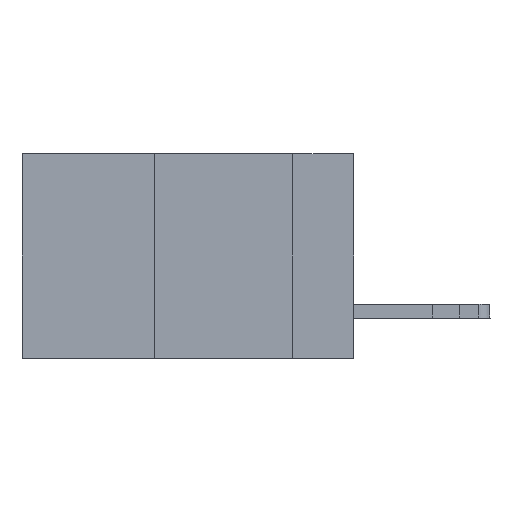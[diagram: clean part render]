
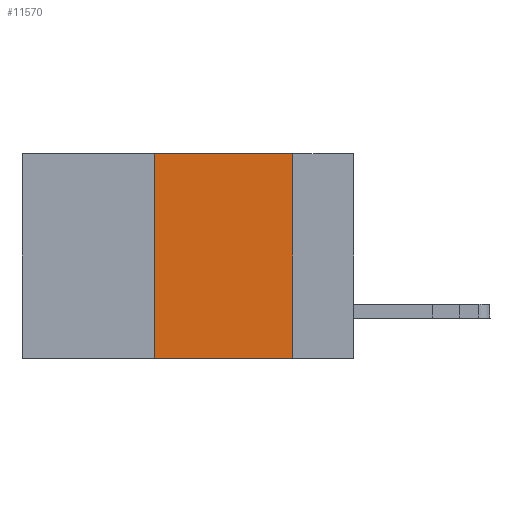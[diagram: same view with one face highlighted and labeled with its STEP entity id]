
A CAD part, left-side view. The second image highlights one B-rep face of the part: STEP entity #11570.
In plain terms, the highlighted planar face has unit normal (-1, 0, 0).
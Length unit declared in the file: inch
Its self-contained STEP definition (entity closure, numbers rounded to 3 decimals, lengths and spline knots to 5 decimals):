
#340 = CARTESIAN_POINT ( 'NONE',  ( 0., 0.36, 0. ) ) ;
#1630 = CARTESIAN_POINT ( 'NONE',  ( 0., 0.6, -0.37 ) ) ;
#2541 = CARTESIAN_POINT ( 'NONE',  ( 0., 0.36, -0.37 ) ) ;
#2728 = LINE ( 'NONE', #13764, #15780 ) ;
#3013 = DIRECTION ( 'NONE',  ( 0., -1., 0. ) ) ;
#3130 = LINE ( 'NONE', #1630, #9951 ) ;
#3228 = EDGE_CURVE ( 'NONE', #16537, #3969, #11790, .T. ) ;
#3969 = VERTEX_POINT ( 'NONE', #9981 ) ;
#5041 = AXIS2_PLACEMENT_3D ( 'NONE', #12373, #7009, #16317 ) ;
#5202 = ORIENTED_EDGE ( 'NONE', *, *, #9447, .F. ) ;
#6876 = CARTESIAN_POINT ( 'NONE',  ( 0., 0.6, 0. ) ) ;
#7009 = DIRECTION ( 'NONE',  ( 1., 0., 0. ) ) ;
#7068 = DIRECTION ( 'NONE',  ( 0., 0., -1. ) ) ;
#7165 = EDGE_CURVE ( 'NONE', #3969, #14063, #2728, .T. ) ;
#7179 = ORIENTED_EDGE ( 'NONE', *, *, #3228, .F. ) ;
#8226 = VECTOR ( 'NONE', #12306, 39.37008 ) ;
#8603 = CARTESIAN_POINT ( 'NONE',  ( 0., 0.11, -0.37 ) ) ;
#8669 = VERTEX_POINT ( 'NONE', #2541 ) ;
#9447 = EDGE_CURVE ( 'NONE', #8669, #16537, #13070, .T. ) ;
#9951 = VECTOR ( 'NONE', #3013, 39.37008 ) ;
#9981 = CARTESIAN_POINT ( 'NONE',  ( 0., 0.11, 0. ) ) ;
#11570 = ADVANCED_FACE ( 'NONE', ( #16278 ), #15021, .F. ) ;
#11790 = LINE ( 'NONE', #6876, #8226 ) ;
#12200 = ORIENTED_EDGE ( 'NONE', *, *, #7165, .F. ) ;
#12306 = DIRECTION ( 'NONE',  ( 0., -1., 0. ) ) ;
#12373 = CARTESIAN_POINT ( 'NONE',  ( 0., 0.6, 0. ) ) ;
#12646 = VECTOR ( 'NONE', #15231, 39.37008 ) ;
#13070 = LINE ( 'NONE', #340, #12646 ) ;
#13764 = CARTESIAN_POINT ( 'NONE',  ( 0., 0.11, 0. ) ) ;
#14063 = VERTEX_POINT ( 'NONE', #8603 ) ;
#14079 = CARTESIAN_POINT ( 'NONE',  ( 0., 0.36, 0. ) ) ;
#14658 = ORIENTED_EDGE ( 'NONE', *, *, #16408, .T. ) ;
#15021 = PLANE ( 'NONE',  #5041 ) ;
#15231 = DIRECTION ( 'NONE',  ( 0., 0., 1. ) ) ;
#15780 = VECTOR ( 'NONE', #7068, 39.37008 ) ;
#16278 = FACE_OUTER_BOUND ( 'NONE', #16725, .T. ) ;
#16317 = DIRECTION ( 'NONE',  ( 0., 0., -1. ) ) ;
#16408 = EDGE_CURVE ( 'NONE', #8669, #14063, #3130, .T. ) ;
#16537 = VERTEX_POINT ( 'NONE', #14079 ) ;
#16725 = EDGE_LOOP ( 'NONE', ( #12200, #7179, #5202, #14658 ) ) ;
